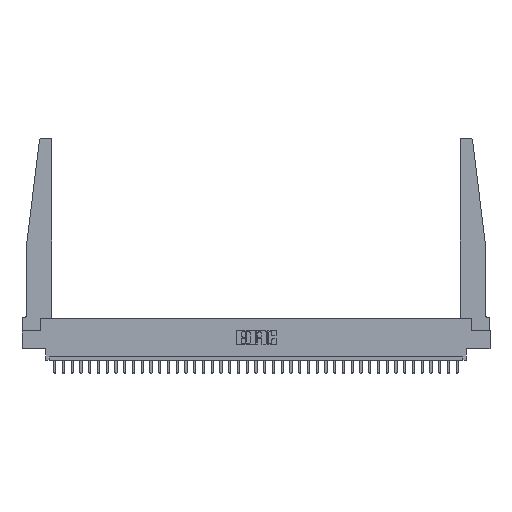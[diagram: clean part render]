
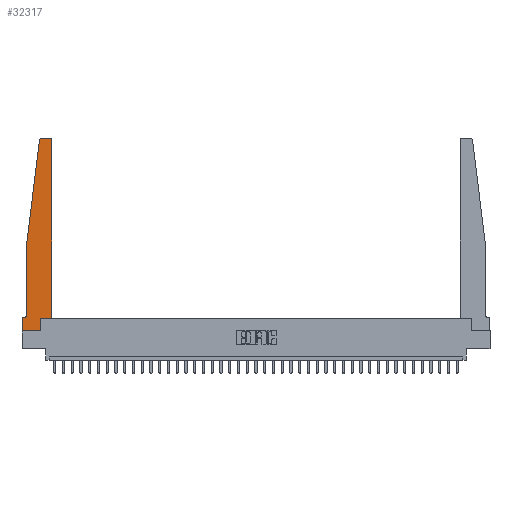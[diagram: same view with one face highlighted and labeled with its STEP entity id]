
A CAD part, top view. The second image highlights one B-rep face of the part: STEP entity #32317.
In plain terms, the highlighted planar face has unit normal (0, 0, 1).
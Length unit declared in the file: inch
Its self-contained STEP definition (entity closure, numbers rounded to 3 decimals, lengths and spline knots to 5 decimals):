
#387 = EDGE_CURVE ( 'NONE', #32852, #16850, #13592, .T. ) ;
#431 = DIRECTION ( 'NONE',  ( 1., 0., 0. ) ) ;
#1097 = LINE ( 'NONE', #29611, #25784 ) ;
#1472 = LINE ( 'NONE', #11043, #28177 ) ;
#1651 = LINE ( 'NONE', #13309, #9343 ) ;
#1993 = CARTESIAN_POINT ( 'NONE',  ( 0.2605, 0.18, 0.37 ) ) ;
#2108 = ORIENTED_EDGE ( 'NONE', *, *, #25411, .T. ) ;
#2404 = DIRECTION ( 'NONE',  ( 1., 0., 0. ) ) ;
#2697 = CARTESIAN_POINT ( 'NONE',  ( 0.24675, 2.72367, 0.37 ) ) ;
#2868 = CARTESIAN_POINT ( 'NONE',  ( 0.395, 2.75, 0.37 ) ) ;
#2876 = ORIENTED_EDGE ( 'NONE', *, *, #26383, .T. ) ;
#3237 = AXIS2_PLACEMENT_3D ( 'NONE', #29648, #3787, #6367 ) ;
#3496 = LINE ( 'NONE', #13273, #13957 ) ;
#3787 = DIRECTION ( 'NONE',  ( 0., 0., 1. ) ) ;
#4139 = ORIENTED_EDGE ( 'NONE', *, *, #19554, .T. ) ;
#4251 = AXIS2_PLACEMENT_3D ( 'NONE', #15446, #10008, #28118 ) ;
#4464 = VERTEX_POINT ( 'NONE', #1993 ) ;
#4795 = CIRCLE ( 'NONE', #3237, 0.03 ) ;
#5249 = DIRECTION ( 'NONE',  ( 0., 0., 1. ) ) ;
#5979 = EDGE_CURVE ( 'NONE', #22196, #25824, #3496, .T. ) ;
#6367 = DIRECTION ( 'NONE',  ( 1., 0., 0. ) ) ;
#6637 = CARTESIAN_POINT ( 'NONE',  ( 0.015, 0.1875, 0.37 ) ) ;
#7004 = EDGE_CURVE ( 'NONE', #18426, #32852, #26883, .T. ) ;
#7269 = CARTESIAN_POINT ( 'NONE',  ( 0.425, 0.18, 0.37 ) ) ;
#7432 = CARTESIAN_POINT ( 'NONE',  ( 0.065, 1.25, 0.37 ) ) ;
#8052 = VERTEX_POINT ( 'NONE', #14917 ) ;
#8091 = DIRECTION ( 'NONE',  ( -1., 0., 0. ) ) ;
#9221 = DIRECTION ( 'NONE',  ( -1., 0., 0. ) ) ;
#9343 = VECTOR ( 'NONE', #431, 39.37008 ) ;
#10008 = DIRECTION ( 'NONE',  ( 0., 0., 1. ) ) ;
#11043 = CARTESIAN_POINT ( 'NONE',  ( 0.2605, 0.18, 0.37 ) ) ;
#11349 = EDGE_LOOP ( 'NONE', ( #22635, #2108, #19724, #4139, #27287, #23066, #12981, #24975, #2876, #24158, #16005, #25339 ) ) ;
#11707 = EDGE_CURVE ( 'NONE', #16850, #33160, #1097, .T. ) ;
#12981 = ORIENTED_EDGE ( 'NONE', *, *, #25377, .T. ) ;
#13273 = CARTESIAN_POINT ( 'NONE',  ( 0.065, 0.1875, 0.37 ) ) ;
#13309 = CARTESIAN_POINT ( 'NONE',  ( 0.425, 0.18, 0.37 ) ) ;
#13592 = CIRCLE ( 'NONE', #4251, 0.03 ) ;
#13943 = LINE ( 'NONE', #16161, #24482 ) ;
#13957 = VECTOR ( 'NONE', #8091, 39.37008 ) ;
#14365 = DIRECTION ( 'NONE',  ( 0., -1., 0. ) ) ;
#14917 = CARTESIAN_POINT ( 'NONE',  ( 0.065, 0.2375, 0.37 ) ) ;
#15187 = PLANE ( 'NONE',  #32839 ) ;
#15446 = CARTESIAN_POINT ( 'NONE',  ( 0.395, 2.72, 0.37 ) ) ;
#15462 = DIRECTION ( 'NONE',  ( -0.122, -0.992, 0. ) ) ;
#15472 = VERTEX_POINT ( 'NONE', #2697 ) ;
#16005 = ORIENTED_EDGE ( 'NONE', *, *, #7004, .T. ) ;
#16047 = DIRECTION ( 'NONE',  ( 1., 0., 0. ) ) ;
#16161 = CARTESIAN_POINT ( 'NONE',  ( 0., 0., 0.37 ) ) ;
#16244 = DIRECTION ( 'NONE',  ( 0., 1., 0. ) ) ;
#16682 = VERTEX_POINT ( 'NONE', #21816 ) ;
#16850 = VERTEX_POINT ( 'NONE', #2868 ) ;
#17929 = CIRCLE ( 'NONE', #21474, 0.05 ) ;
#17970 = DIRECTION ( 'NONE',  ( 0., 1., 0. ) ) ;
#18160 = EDGE_CURVE ( 'NONE', #8052, #22196, #17929, .T. ) ;
#18426 = VERTEX_POINT ( 'NONE', #7269 ) ;
#19164 = EDGE_CURVE ( 'NONE', #4464, #18426, #1651, .T. ) ;
#19349 = DIRECTION ( 'NONE',  ( -1., 0., 0. ) ) ;
#19554 = EDGE_CURVE ( 'NONE', #27366, #8052, #27140, .T. ) ;
#19724 = ORIENTED_EDGE ( 'NONE', *, *, #24352, .T. ) ;
#20697 = CARTESIAN_POINT ( 'NONE',  ( 0., 0.1875, 0.37 ) ) ;
#21314 = FACE_OUTER_BOUND ( 'NONE', #11349, .T. ) ;
#21327 = LINE ( 'NONE', #29877, #31497 ) ;
#21458 = CARTESIAN_POINT ( 'NONE',  ( 0.065, 1.25, 0.37 ) ) ;
#21474 = AXIS2_PLACEMENT_3D ( 'NONE', #32731, #27209, #9221 ) ;
#21816 = CARTESIAN_POINT ( 'NONE',  ( 0.2605, 0., 0.37 ) ) ;
#22196 = VERTEX_POINT ( 'NONE', #6637 ) ;
#22249 = CARTESIAN_POINT ( 'NONE',  ( 0.425, 0.18, 0.37 ) ) ;
#22635 = ORIENTED_EDGE ( 'NONE', *, *, #11707, .T. ) ;
#23056 = CARTESIAN_POINT ( 'NONE',  ( 0.27653, 2.75, 0.37 ) ) ;
#23066 = ORIENTED_EDGE ( 'NONE', *, *, #5979, .T. ) ;
#23093 = VECTOR ( 'NONE', #29391, 39.37008 ) ;
#23515 = CARTESIAN_POINT ( 'NONE',  ( 0., 0.1875, 0.37 ) ) ;
#24158 = ORIENTED_EDGE ( 'NONE', *, *, #19164, .T. ) ;
#24352 = EDGE_CURVE ( 'NONE', #15472, #27366, #28325, .T. ) ;
#24439 = CARTESIAN_POINT ( 'NONE',  ( 0.425, 2.72, 0.37 ) ) ;
#24482 = VECTOR ( 'NONE', #16047, 39.37008 ) ;
#24910 = VERTEX_POINT ( 'NONE', #28323 ) ;
#24975 = ORIENTED_EDGE ( 'NONE', *, *, #33417, .T. ) ;
#25339 = ORIENTED_EDGE ( 'NONE', *, *, #387, .T. ) ;
#25377 = EDGE_CURVE ( 'NONE', #25824, #24910, #21327, .T. ) ;
#25411 = EDGE_CURVE ( 'NONE', #33160, #15472, #4795, .T. ) ;
#25784 = VECTOR ( 'NONE', #19349, 39.37008 ) ;
#25824 = VERTEX_POINT ( 'NONE', #23515 ) ;
#26383 = EDGE_CURVE ( 'NONE', #16682, #4464, #1472, .T. ) ;
#26883 = LINE ( 'NONE', #22249, #32941 ) ;
#27140 = LINE ( 'NONE', #21458, #23093 ) ;
#27209 = DIRECTION ( 'NONE',  ( 0., 0., -1. ) ) ;
#27287 = ORIENTED_EDGE ( 'NONE', *, *, #18160, .T. ) ;
#27349 = CARTESIAN_POINT ( 'NONE',  ( 0.065, 1.25, 0.37 ) ) ;
#27366 = VERTEX_POINT ( 'NONE', #27349 ) ;
#28118 = DIRECTION ( 'NONE',  ( 1., 0., 0. ) ) ;
#28177 = VECTOR ( 'NONE', #16244, 39.37008 ) ;
#28323 = CARTESIAN_POINT ( 'NONE',  ( 0., 0., 0.37 ) ) ;
#28325 = LINE ( 'NONE', #7432, #32806 ) ;
#29391 = DIRECTION ( 'NONE',  ( 0., -1., 0. ) ) ;
#29611 = CARTESIAN_POINT ( 'NONE',  ( 0.25, 2.75, 0.37 ) ) ;
#29648 = CARTESIAN_POINT ( 'NONE',  ( 0.27653, 2.72, 0.37 ) ) ;
#29877 = CARTESIAN_POINT ( 'NONE',  ( 0., 0., 0.37 ) ) ;
#31497 = VECTOR ( 'NONE', #14365, 39.37008 ) ;
#32317 = ADVANCED_FACE ( 'NONE', ( #21314 ), #15187, .T. ) ;
#32731 = CARTESIAN_POINT ( 'NONE',  ( 0.015, 0.2375, 0.37 ) ) ;
#32806 = VECTOR ( 'NONE', #15462, 39.37008 ) ;
#32839 = AXIS2_PLACEMENT_3D ( 'NONE', #20697, #5249, #2404 ) ;
#32852 = VERTEX_POINT ( 'NONE', #24439 ) ;
#32941 = VECTOR ( 'NONE', #17970, 39.37008 ) ;
#33160 = VERTEX_POINT ( 'NONE', #23056 ) ;
#33417 = EDGE_CURVE ( 'NONE', #24910, #16682, #13943, .T. ) ;
